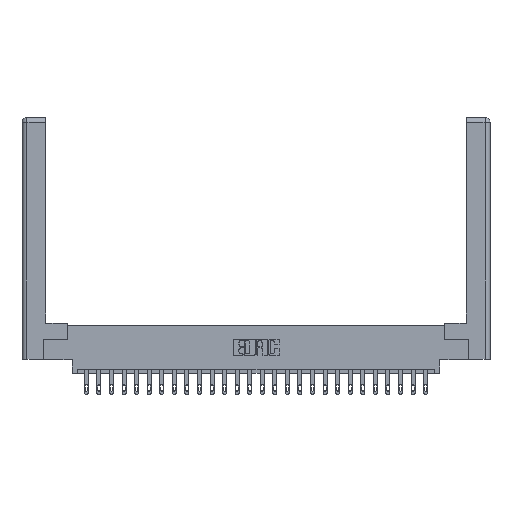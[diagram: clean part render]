
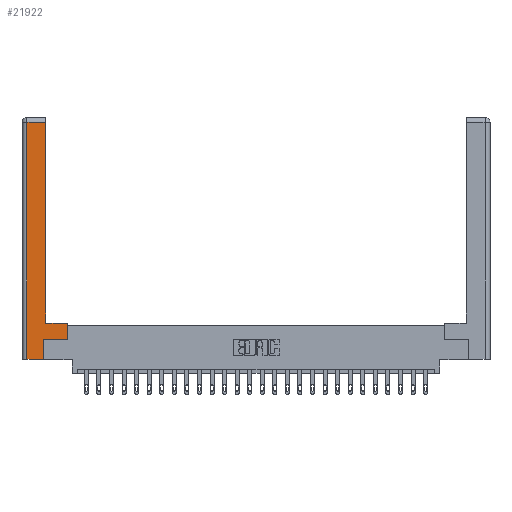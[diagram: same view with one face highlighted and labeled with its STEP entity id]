
A CAD part, top view. The second image highlights one B-rep face of the part: STEP entity #21922.
In plain terms, the highlighted planar face has unit normal (0, 0, 1).
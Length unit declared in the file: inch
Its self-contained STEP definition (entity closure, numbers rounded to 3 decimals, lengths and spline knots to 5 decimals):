
#244 = CARTESIAN_POINT ( 'NONE',  ( 0.565, 0.245, 0. ) ) ;
#306 = LINE ( 'NONE', #22298, #22511 ) ;
#1039 = VECTOR ( 'NONE', #5976, 39.37008 ) ;
#1366 = VERTEX_POINT ( 'NONE', #19964 ) ;
#1664 = LINE ( 'NONE', #4418, #3562 ) ;
#2323 = VECTOR ( 'NONE', #12063, 39.37008 ) ;
#2412 = CARTESIAN_POINT ( 'NONE',  ( 0.295, 2.94, 0. ) ) ;
#3562 = VECTOR ( 'NONE', #22725, 39.37008 ) ;
#4418 = CARTESIAN_POINT ( 'NONE',  ( 0.0615, 2.94, 0. ) ) ;
#4926 = ORIENTED_EDGE ( 'NONE', *, *, #12547, .T. ) ;
#4931 = VERTEX_POINT ( 'NONE', #23645 ) ;
#5403 = VERTEX_POINT ( 'NONE', #24715 ) ;
#5976 = DIRECTION ( 'NONE',  ( 1., 0., 0. ) ) ;
#6150 = EDGE_CURVE ( 'NONE', #20068, #1366, #1664, .T. ) ;
#6297 = CARTESIAN_POINT ( 'NONE',  ( 0.265, 0., 0. ) ) ;
#6946 = CARTESIAN_POINT ( 'NONE',  ( 0., 0., 0. ) ) ;
#6993 = CARTESIAN_POINT ( 'NONE',  ( 0.295, 0.45, 0. ) ) ;
#7159 = CARTESIAN_POINT ( 'NONE',  ( 0.565, 0.45, 0. ) ) ;
#8034 = DIRECTION ( 'NONE',  ( 0., -1., 0. ) ) ;
#8114 = VERTEX_POINT ( 'NONE', #7159 ) ;
#8847 = PLANE ( 'NONE',  #17336 ) ;
#9220 = LINE ( 'NONE', #11786, #25046 ) ;
#9271 = CARTESIAN_POINT ( 'NONE',  ( 0.565, 0.45, 0. ) ) ;
#9553 = ORIENTED_EDGE ( 'NONE', *, *, #19458, .T. ) ;
#10914 = DIRECTION ( 'NONE',  ( 0., 0., -1. ) ) ;
#10948 = ORIENTED_EDGE ( 'NONE', *, *, #20126, .T. ) ;
#11243 = ORIENTED_EDGE ( 'NONE', *, *, #12534, .T. ) ;
#11482 = DIRECTION ( 'NONE',  ( 0., 1., 0. ) ) ;
#11786 = CARTESIAN_POINT ( 'NONE',  ( 0.0615, 0., 0. ) ) ;
#12063 = DIRECTION ( 'NONE',  ( -1., 0., 0. ) ) ;
#12534 = EDGE_CURVE ( 'NONE', #8114, #15565, #21341, .T. ) ;
#12547 = EDGE_CURVE ( 'NONE', #4931, #23630, #12806, .T. ) ;
#12639 = DIRECTION ( 'NONE',  ( 0., 1., 0. ) ) ;
#12806 = LINE ( 'NONE', #14268, #1039 ) ;
#14268 = CARTESIAN_POINT ( 'NONE',  ( 0.565, 0.245, 0. ) ) ;
#14672 = DIRECTION ( 'NONE',  ( 1., 0., 0. ) ) ;
#15204 = LINE ( 'NONE', #9271, #23120 ) ;
#15416 = EDGE_CURVE ( 'NONE', #20985, #5403, #23082, .T. ) ;
#15565 = VERTEX_POINT ( 'NONE', #6993 ) ;
#17336 = AXIS2_PLACEMENT_3D ( 'NONE', #6946, #10914, #24875 ) ;
#18063 = CARTESIAN_POINT ( 'NONE',  ( 0.295, 0.45, 0. ) ) ;
#18970 = VECTOR ( 'NONE', #14672, 39.37008 ) ;
#19270 = CARTESIAN_POINT ( 'NONE',  ( 0.0615, 0., 0. ) ) ;
#19272 = VECTOR ( 'NONE', #11482, 39.37008 ) ;
#19458 = EDGE_CURVE ( 'NONE', #1366, #20985, #9220, .T. ) ;
#19858 = ORIENTED_EDGE ( 'NONE', *, *, #6150, .T. ) ;
#19964 = CARTESIAN_POINT ( 'NONE',  ( 0.0615, 2.94, 0. ) ) ;
#20068 = VERTEX_POINT ( 'NONE', #2412 ) ;
#20122 = EDGE_CURVE ( 'NONE', #5403, #4931, #306, .T. ) ;
#20126 = EDGE_CURVE ( 'NONE', #23630, #8114, #15204, .T. ) ;
#20552 = LINE ( 'NONE', #25875, #19272 ) ;
#20985 = VERTEX_POINT ( 'NONE', #19270 ) ;
#21085 = EDGE_CURVE ( 'NONE', #15565, #20068, #20552, .T. ) ;
#21341 = LINE ( 'NONE', #18063, #2323 ) ;
#21922 = ADVANCED_FACE ( 'NONE', ( #25853 ), #8847, .F. ) ;
#22298 = CARTESIAN_POINT ( 'NONE',  ( 0.265, 0.245, 0. ) ) ;
#22498 = DIRECTION ( 'NONE',  ( 0., 1., 0. ) ) ;
#22511 = VECTOR ( 'NONE', #22498, 39.37008 ) ;
#22725 = DIRECTION ( 'NONE',  ( -1., 0., 0. ) ) ;
#22971 = ORIENTED_EDGE ( 'NONE', *, *, #20122, .T. ) ;
#23082 = LINE ( 'NONE', #6297, #18970 ) ;
#23120 = VECTOR ( 'NONE', #12639, 39.37008 ) ;
#23630 = VERTEX_POINT ( 'NONE', #244 ) ;
#23645 = CARTESIAN_POINT ( 'NONE',  ( 0.265, 0.245, 0. ) ) ;
#24715 = CARTESIAN_POINT ( 'NONE',  ( 0.265, 0., 0. ) ) ;
#24875 = DIRECTION ( 'NONE',  ( -1., 0., 0. ) ) ;
#24977 = EDGE_LOOP ( 'NONE', ( #25060, #19858, #9553, #25323, #22971, #4926, #10948, #11243 ) ) ;
#25046 = VECTOR ( 'NONE', #8034, 39.37008 ) ;
#25060 = ORIENTED_EDGE ( 'NONE', *, *, #21085, .T. ) ;
#25323 = ORIENTED_EDGE ( 'NONE', *, *, #15416, .T. ) ;
#25853 = FACE_OUTER_BOUND ( 'NONE', #24977, .T. ) ;
#25875 = CARTESIAN_POINT ( 'NONE',  ( 0.295, 3., 0. ) ) ;
